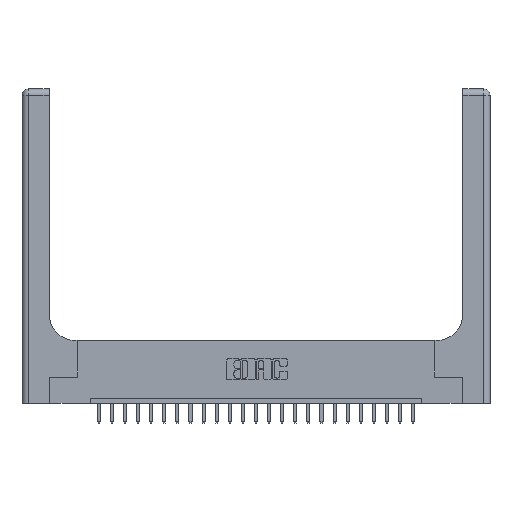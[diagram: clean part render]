
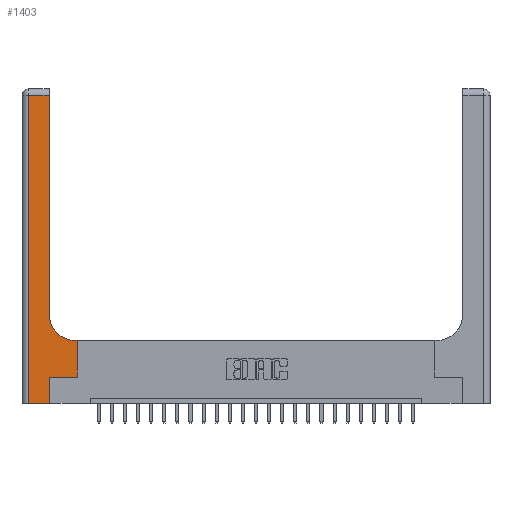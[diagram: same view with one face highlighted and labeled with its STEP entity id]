
A CAD part, top view. The second image highlights one B-rep face of the part: STEP entity #1403.
In plain terms, the highlighted planar face has unit normal (0, 0, 1).
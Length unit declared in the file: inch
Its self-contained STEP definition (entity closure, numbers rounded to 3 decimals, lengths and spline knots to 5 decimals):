
#20 = DIRECTION ( 'NONE',  ( -1., 0., 0. ) ) ;
#570 = ORIENTED_EDGE ( 'NONE', *, *, #3008, .T. ) ;
#816 = ORIENTED_EDGE ( 'NONE', *, *, #13354, .T. ) ;
#819 = CARTESIAN_POINT ( 'NONE',  ( 0.51, 0.85, 0.37 ) ) ;
#1403 = ADVANCED_FACE ( 'NONE', ( #2295 ), #17823, .F. ) ;
#1429 = VECTOR ( 'NONE', #16831, 39.37008 ) ;
#2057 = LINE ( 'NONE', #22333, #17998 ) ;
#2295 = FACE_OUTER_BOUND ( 'NONE', #7897, .T. ) ;
#2315 = ORIENTED_EDGE ( 'NONE', *, *, #22570, .T. ) ;
#2877 = EDGE_CURVE ( 'NONE', #14045, #3003, #15671, .T. ) ;
#3003 = VERTEX_POINT ( 'NONE', #18466 ) ;
#3008 = EDGE_CURVE ( 'NONE', #11551, #20269, #10030, .T. ) ;
#4487 = ORIENTED_EDGE ( 'NONE', *, *, #13171, .T. ) ;
#4517 = AXIS2_PLACEMENT_3D ( 'NONE', #819, #22275, #16857 ) ;
#4859 = LINE ( 'NONE', #7107, #7938 ) ;
#5008 = ORIENTED_EDGE ( 'NONE', *, *, #19764, .T. ) ;
#6073 = EDGE_CURVE ( 'NONE', #13365, #17656, #2057, .T. ) ;
#6520 = CARTESIAN_POINT ( 'NONE',  ( 0., 2.94, 0.37 ) ) ;
#6940 = CARTESIAN_POINT ( 'NONE',  ( 0.528, 0.6, 0.37 ) ) ;
#6951 = VECTOR ( 'NONE', #8022, 39.37008 ) ;
#7107 = CARTESIAN_POINT ( 'NONE',  ( 0.26, 3., 0.37 ) ) ;
#7897 = EDGE_LOOP ( 'NONE', ( #19808, #570, #4487, #16690, #10240, #2315, #816, #16648, #5008 ) ) ;
#7938 = VECTOR ( 'NONE', #15788, 39.37008 ) ;
#7974 = CARTESIAN_POINT ( 'NONE',  ( 0.06, 0., 0.37 ) ) ;
#8022 = DIRECTION ( 'NONE',  ( 0., 1., 0. ) ) ;
#8755 = CARTESIAN_POINT ( 'NONE',  ( 0., 3., 0.37 ) ) ;
#8913 = CARTESIAN_POINT ( 'NONE',  ( 0.06, 2.94, 0.37 ) ) ;
#8942 = DIRECTION ( 'NONE',  ( 0., 1., 0. ) ) ;
#9387 = VECTOR ( 'NONE', #13250, 39.37008 ) ;
#9626 = CARTESIAN_POINT ( 'NONE',  ( 0.06, 3., 0.37 ) ) ;
#9659 = CARTESIAN_POINT ( 'NONE',  ( 0.528, 0.25, 0.37 ) ) ;
#9660 = CARTESIAN_POINT ( 'NONE',  ( 0.265, 0., 0.37 ) ) ;
#10030 = LINE ( 'NONE', #6520, #19243 ) ;
#10103 = LINE ( 'NONE', #9626, #1429 ) ;
#10165 = CARTESIAN_POINT ( 'NONE',  ( 0.51, 0.6, 0.37 ) ) ;
#10240 = ORIENTED_EDGE ( 'NONE', *, *, #16965, .T. ) ;
#11108 = EDGE_CURVE ( 'NONE', #16935, #11551, #4859, .T. ) ;
#11129 = VERTEX_POINT ( 'NONE', #19408 ) ;
#11551 = VERTEX_POINT ( 'NONE', #19229 ) ;
#12708 = VERTEX_POINT ( 'NONE', #9659 ) ;
#13051 = LINE ( 'NONE', #16757, #9387 ) ;
#13111 = AXIS2_PLACEMENT_3D ( 'NONE', #8755, #19575, #21217 ) ;
#13171 = EDGE_CURVE ( 'NONE', #20269, #14045, #10103, .T. ) ;
#13250 = DIRECTION ( 'NONE',  ( 1., 0., 0. ) ) ;
#13354 = EDGE_CURVE ( 'NONE', #12708, #13365, #19819, .T. ) ;
#13365 = VERTEX_POINT ( 'NONE', #6940 ) ;
#13432 = VECTOR ( 'NONE', #8942, 39.37008 ) ;
#13954 = LINE ( 'NONE', #9660, #6951 ) ;
#14045 = VERTEX_POINT ( 'NONE', #7974 ) ;
#15671 = LINE ( 'NONE', #19464, #18702 ) ;
#15788 = DIRECTION ( 'NONE',  ( 0., 1., 0. ) ) ;
#16648 = ORIENTED_EDGE ( 'NONE', *, *, #6073, .T. ) ;
#16685 = DIRECTION ( 'NONE',  ( -1., 0., 0. ) ) ;
#16690 = ORIENTED_EDGE ( 'NONE', *, *, #2877, .T. ) ;
#16757 = CARTESIAN_POINT ( 'NONE',  ( 0.265, 0.25, 0.37 ) ) ;
#16831 = DIRECTION ( 'NONE',  ( 0., -1., 0. ) ) ;
#16857 = DIRECTION ( 'NONE',  ( 1., 0., 0. ) ) ;
#16935 = VERTEX_POINT ( 'NONE', #18546 ) ;
#16965 = EDGE_CURVE ( 'NONE', #3003, #11129, #13954, .T. ) ;
#17656 = VERTEX_POINT ( 'NONE', #10165 ) ;
#17823 = PLANE ( 'NONE',  #13111 ) ;
#17998 = VECTOR ( 'NONE', #16685, 39.37008 ) ;
#18466 = CARTESIAN_POINT ( 'NONE',  ( 0.265, 0., 0.37 ) ) ;
#18546 = CARTESIAN_POINT ( 'NONE',  ( 0.26, 0.85, 0.37 ) ) ;
#18702 = VECTOR ( 'NONE', #19388, 39.37008 ) ;
#19105 = CIRCLE ( 'NONE', #4517, 0.25 ) ;
#19229 = CARTESIAN_POINT ( 'NONE',  ( 0.26, 2.94, 0.37 ) ) ;
#19243 = VECTOR ( 'NONE', #20, 39.37008 ) ;
#19388 = DIRECTION ( 'NONE',  ( 1., 0., 0. ) ) ;
#19408 = CARTESIAN_POINT ( 'NONE',  ( 0.265, 0.25, 0.37 ) ) ;
#19464 = CARTESIAN_POINT ( 'NONE',  ( 0., 0., 0.37 ) ) ;
#19575 = DIRECTION ( 'NONE',  ( 0., 0., -1. ) ) ;
#19764 = EDGE_CURVE ( 'NONE', #17656, #16935, #19105, .T. ) ;
#19808 = ORIENTED_EDGE ( 'NONE', *, *, #11108, .T. ) ;
#19819 = LINE ( 'NONE', #21332, #13432 ) ;
#20269 = VERTEX_POINT ( 'NONE', #8913 ) ;
#21217 = DIRECTION ( 'NONE',  ( -1., 0., 0. ) ) ;
#21332 = CARTESIAN_POINT ( 'NONE',  ( 0.528, 0.25, 0.37 ) ) ;
#22275 = DIRECTION ( 'NONE',  ( 0., 0., -1. ) ) ;
#22333 = CARTESIAN_POINT ( 'NONE',  ( 0.26, 0.6, 0.37 ) ) ;
#22570 = EDGE_CURVE ( 'NONE', #11129, #12708, #13051, .T. ) ;
